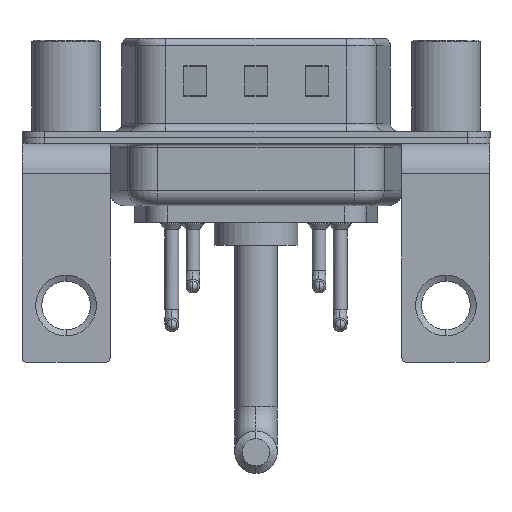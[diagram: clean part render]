
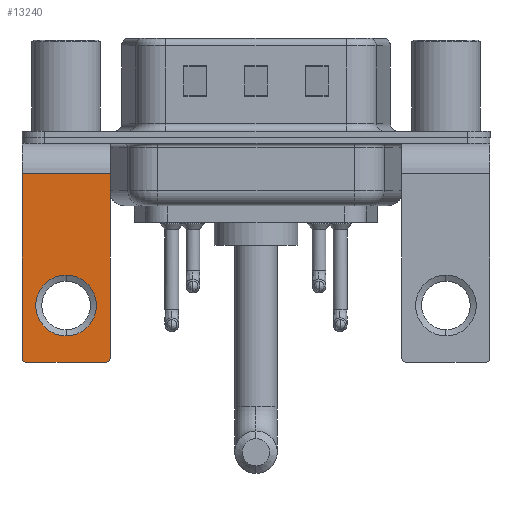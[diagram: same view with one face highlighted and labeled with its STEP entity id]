
A CAD part, front view. The second image highlights one B-rep face of the part: STEP entity #13240.
In plain terms, the highlighted planar face has unit normal (0, -1, 0).
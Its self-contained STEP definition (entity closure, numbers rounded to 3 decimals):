
#273 = ORIENTED_EDGE ( 'NONE', *, *, #19880, .T. ) ;
#370 = VECTOR ( 'NONE', #19729, 1000. ) ;
#533 = DIRECTION ( 'NONE',  ( 0., 0., 1. ) ) ;
#2225 = ORIENTED_EDGE ( 'NONE', *, *, #8659, .T. ) ;
#2461 = CIRCLE ( 'NONE', #14426, 0.25 ) ;
#3024 = CARTESIAN_POINT ( 'NONE',  ( 2.65, -6.25, -14.55 ) ) ;
#4540 = VERTEX_POINT ( 'NONE', #9449 ) ;
#4679 = DIRECTION ( 'NONE',  ( 0., 0., 1. ) ) ;
#4795 = VERTEX_POINT ( 'NONE', #11653 ) ;
#5119 = DIRECTION ( 'NONE',  ( 0., -1., 0. ) ) ;
#5432 = CARTESIAN_POINT ( 'NONE',  ( 2.9, -6.25, -14.55 ) ) ;
#5615 = EDGE_CURVE ( 'NONE', #4795, #9377, #6143, .T. ) ;
#6005 = CARTESIAN_POINT ( 'NONE',  ( 2.9, -6.25, -2.4 ) ) ;
#6097 = CARTESIAN_POINT ( 'NONE',  ( 0., -6.25, -11.07 ) ) ;
#6143 = LINE ( 'NONE', #21417, #12522 ) ;
#6207 = DIRECTION ( 'NONE',  ( 0., 1., 0. ) ) ;
#6251 = DIRECTION ( 'NONE',  ( 0., 0., -1. ) ) ;
#6542 = ORIENTED_EDGE ( 'NONE', *, *, #18960, .T. ) ;
#6658 = DIRECTION ( 'NONE',  ( -1., 0., 0. ) ) ;
#7000 = EDGE_LOOP ( 'NONE', ( #6542, #2225 ) ) ;
#7057 = AXIS2_PLACEMENT_3D ( 'NONE', #6005, #9441, #4679 ) ;
#7764 = CARTESIAN_POINT ( 'NONE',  ( 2.9, -6.25, -2.4 ) ) ;
#7973 = DIRECTION ( 'NONE',  ( 0., 0., 1. ) ) ;
#8077 = VECTOR ( 'NONE', #6658, 1000. ) ;
#8659 = EDGE_CURVE ( 'NONE', #16039, #4540, #21667, .T. ) ;
#9050 = VERTEX_POINT ( 'NONE', #18817 ) ;
#9155 = DIRECTION ( 'NONE',  ( 0., -1., 0. ) ) ;
#9289 = LINE ( 'NONE', #14358, #15467 ) ;
#9377 = VERTEX_POINT ( 'NONE', #13142 ) ;
#9441 = DIRECTION ( 'NONE',  ( 0., 1., 0. ) ) ;
#9449 = CARTESIAN_POINT ( 'NONE',  ( 0., -6.25, -13.07 ) ) ;
#10203 = CARTESIAN_POINT ( 'NONE',  ( -2.65, -6.25, -14.55 ) ) ;
#11441 = AXIS2_PLACEMENT_3D ( 'NONE', #6097, #6207, #17939 ) ;
#11534 = CARTESIAN_POINT ( 'NONE',  ( -2.65, -6.25, -14.8 ) ) ;
#11630 = CARTESIAN_POINT ( 'NONE',  ( 2.65, -6.25, -14.8 ) ) ;
#11653 = CARTESIAN_POINT ( 'NONE',  ( -2.9, -6.25, -2.4 ) ) ;
#12162 = ORIENTED_EDGE ( 'NONE', *, *, #16734, .F. ) ;
#12218 = ORIENTED_EDGE ( 'NONE', *, *, #5615, .T. ) ;
#12336 = DIRECTION ( 'NONE',  ( 0., 1., 0. ) ) ;
#12338 = VERTEX_POINT ( 'NONE', #5432 ) ;
#12522 = VECTOR ( 'NONE', #6251, 1000. ) ;
#12845 = ORIENTED_EDGE ( 'NONE', *, *, #18440, .T. ) ;
#12967 = LINE ( 'NONE', #7764, #370 ) ;
#13142 = CARTESIAN_POINT ( 'NONE',  ( -2.9, -6.25, -14.55 ) ) ;
#13240 = ADVANCED_FACE ( 'NONE', ( #19515, #17841 ), #16301, .F. ) ;
#13304 = EDGE_CURVE ( 'NONE', #9050, #12338, #12967, .T. ) ;
#13519 = CARTESIAN_POINT ( 'NONE',  ( 2.9, -6.25, -2.4 ) ) ;
#14358 = CARTESIAN_POINT ( 'NONE',  ( 2.9, -6.25, -14.8 ) ) ;
#14426 = AXIS2_PLACEMENT_3D ( 'NONE', #3024, #5119, #7973 ) ;
#14732 = LINE ( 'NONE', #13519, #8077 ) ;
#15467 = VECTOR ( 'NONE', #21338, 1000. ) ;
#16039 = VERTEX_POINT ( 'NONE', #16767 ) ;
#16301 = PLANE ( 'NONE',  #7057 ) ;
#16513 = CIRCLE ( 'NONE', #18654, 0.25 ) ;
#16734 = EDGE_CURVE ( 'NONE', #18316, #21765, #9289, .T. ) ;
#16745 = ORIENTED_EDGE ( 'NONE', *, *, #19879, .T. ) ;
#16767 = CARTESIAN_POINT ( 'NONE',  ( 0., -6.25, -9.07 ) ) ;
#17246 = CIRCLE ( 'NONE', #17603, 2. ) ;
#17431 = CARTESIAN_POINT ( 'NONE',  ( 0., -6.25, -11.07 ) ) ;
#17603 = AXIS2_PLACEMENT_3D ( 'NONE', #17431, #12336, #20758 ) ;
#17841 = FACE_OUTER_BOUND ( 'NONE', #20724, .T. ) ;
#17939 = DIRECTION ( 'NONE',  ( 0., 0., 1. ) ) ;
#18316 = VERTEX_POINT ( 'NONE', #11630 ) ;
#18440 = EDGE_CURVE ( 'NONE', #9377, #21765, #16513, .T. ) ;
#18654 = AXIS2_PLACEMENT_3D ( 'NONE', #10203, #9155, #533 ) ;
#18817 = CARTESIAN_POINT ( 'NONE',  ( 2.9, -6.25, -2.4 ) ) ;
#18960 = EDGE_CURVE ( 'NONE', #4540, #16039, #17246, .T. ) ;
#19515 = FACE_BOUND ( 'NONE', #7000, .T. ) ;
#19729 = DIRECTION ( 'NONE',  ( 0., 0., -1. ) ) ;
#19879 = EDGE_CURVE ( 'NONE', #18316, #12338, #2461, .T. ) ;
#19880 = EDGE_CURVE ( 'NONE', #9050, #4795, #14732, .T. ) ;
#20724 = EDGE_LOOP ( 'NONE', ( #12218, #12845, #12162, #16745, #21813, #273 ) ) ;
#20758 = DIRECTION ( 'NONE',  ( 0., 0., 1. ) ) ;
#21338 = DIRECTION ( 'NONE',  ( -1., 0., 0. ) ) ;
#21417 = CARTESIAN_POINT ( 'NONE',  ( -2.9, -6.25, -2.4 ) ) ;
#21667 = CIRCLE ( 'NONE', #11441, 2. ) ;
#21765 = VERTEX_POINT ( 'NONE', #11534 ) ;
#21813 = ORIENTED_EDGE ( 'NONE', *, *, #13304, .F. ) ;
